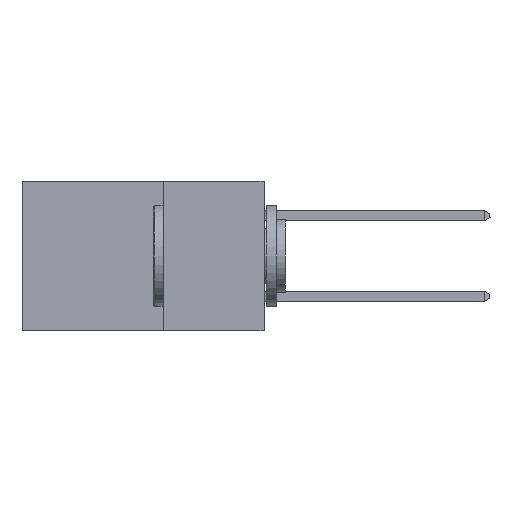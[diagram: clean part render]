
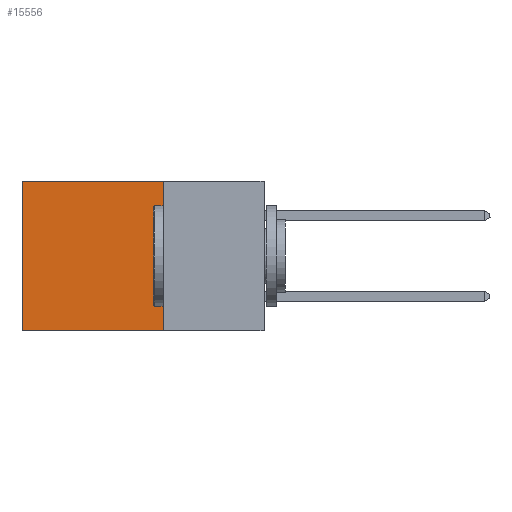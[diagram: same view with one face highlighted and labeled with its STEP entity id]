
A CAD part, left-side view. The second image highlights one B-rep face of the part: STEP entity #15556.
In plain terms, the highlighted planar face has unit normal (-1, 0, 0).
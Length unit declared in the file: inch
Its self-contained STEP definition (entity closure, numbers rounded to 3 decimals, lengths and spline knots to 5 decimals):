
#92 = ORIENTED_EDGE ( 'NONE', *, *, #20685, .F. ) ;
#2319 = CARTESIAN_POINT ( 'NONE',  ( 0.298, 0.25, 0. ) ) ;
#2399 = CARTESIAN_POINT ( 'NONE',  ( 0.298, 0.25, -0.37 ) ) ;
#3228 = ORIENTED_EDGE ( 'NONE', *, *, #16561, .T. ) ;
#3629 = LINE ( 'NONE', #4177, #7638 ) ;
#3965 = DIRECTION ( 'NONE',  ( 0., 0., -1. ) ) ;
#4177 = CARTESIAN_POINT ( 'NONE',  ( 0.298, 0.6, 0. ) ) ;
#5039 = LINE ( 'NONE', #24977, #6708 ) ;
#5144 = AXIS2_PLACEMENT_3D ( 'NONE', #10473, #18878, #3965 ) ;
#5778 = FACE_OUTER_BOUND ( 'NONE', #12926, .T. ) ;
#5821 = ORIENTED_EDGE ( 'NONE', *, *, #8160, .F. ) ;
#6530 = VERTEX_POINT ( 'NONE', #2399 ) ;
#6708 = VECTOR ( 'NONE', #16670, 39.37008 ) ;
#7638 = VECTOR ( 'NONE', #15133, 39.37008 ) ;
#8160 = EDGE_CURVE ( 'NONE', #19788, #6530, #20816, .T. ) ;
#8230 = VECTOR ( 'NONE', #20253, 39.37008 ) ;
#9702 = CARTESIAN_POINT ( 'NONE',  ( 0.298, 0.6, -0.37 ) ) ;
#10473 = CARTESIAN_POINT ( 'NONE',  ( 0.298, 0.25, 0. ) ) ;
#11054 = VERTEX_POINT ( 'NONE', #9702 ) ;
#11525 = VECTOR ( 'NONE', #21080, 39.37008 ) ;
#11746 = ORIENTED_EDGE ( 'NONE', *, *, #25682, .T. ) ;
#12926 = EDGE_LOOP ( 'NONE', ( #11746, #92, #5821, #3228 ) ) ;
#14581 = PLANE ( 'NONE',  #5144 ) ;
#14831 = VERTEX_POINT ( 'NONE', #19695 ) ;
#14985 = CARTESIAN_POINT ( 'NONE',  ( 0.298, 0.25, -0.37 ) ) ;
#15133 = DIRECTION ( 'NONE',  ( 0., 0., -1. ) ) ;
#15556 = ADVANCED_FACE ( 'NONE', ( #5778 ), #14581, .F. ) ;
#16129 = CARTESIAN_POINT ( 'NONE',  ( 0.298, 0.25, 0. ) ) ;
#16561 = EDGE_CURVE ( 'NONE', #19788, #14831, #5039, .T. ) ;
#16670 = DIRECTION ( 'NONE',  ( 0., 1., 0. ) ) ;
#18878 = DIRECTION ( 'NONE',  ( 1., 0., 0. ) ) ;
#19695 = CARTESIAN_POINT ( 'NONE',  ( 0.298, 0.6, 0. ) ) ;
#19788 = VERTEX_POINT ( 'NONE', #2319 ) ;
#20253 = DIRECTION ( 'NONE',  ( 0., 0., -1. ) ) ;
#20685 = EDGE_CURVE ( 'NONE', #6530, #11054, #27104, .T. ) ;
#20816 = LINE ( 'NONE', #16129, #8230 ) ;
#21080 = DIRECTION ( 'NONE',  ( 0., 1., 0. ) ) ;
#24977 = CARTESIAN_POINT ( 'NONE',  ( 0.298, 0.25, 0. ) ) ;
#25682 = EDGE_CURVE ( 'NONE', #14831, #11054, #3629, .T. ) ;
#27104 = LINE ( 'NONE', #14985, #11525 ) ;
